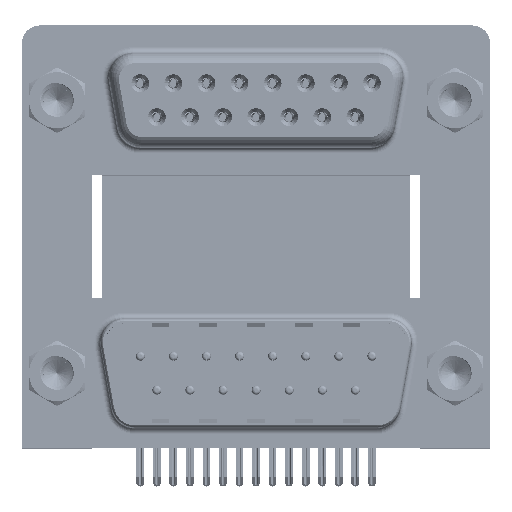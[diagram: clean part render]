
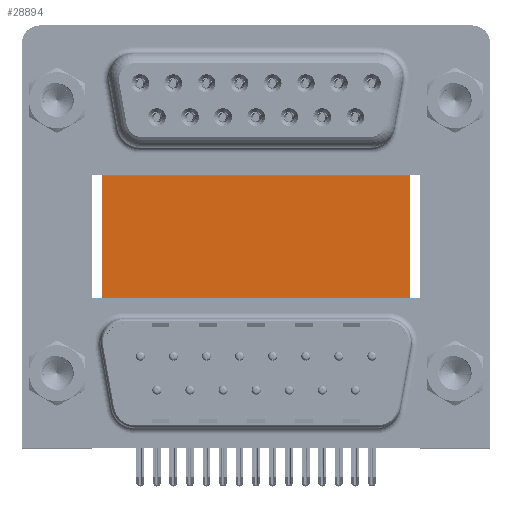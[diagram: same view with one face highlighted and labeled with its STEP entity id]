
A CAD part, top view. The second image highlights one B-rep face of the part: STEP entity #28894.
In plain terms, the highlighted planar face has unit normal (0, 0, 1).
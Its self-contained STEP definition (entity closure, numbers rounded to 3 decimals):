
#5209 = ORIENTED_EDGE ( 'NONE', *, *, #30628, .T. ) ;
#8389 = DIRECTION ( 'NONE',  ( 1., 0., 0. ) ) ;
#11721 = DIRECTION ( 'NONE',  ( 0., 0., -1. ) ) ;
#14759 = VECTOR ( 'NONE', #8389, 1000. ) ;
#15286 = EDGE_CURVE ( 'NONE', #41101, #31572, #44285, .T. ) ;
#15950 = VECTOR ( 'NONE', #24155, 1000. ) ;
#16195 = CARTESIAN_POINT ( 'NONE',  ( 29.58, -3.735, -12. ) ) ;
#16615 = LINE ( 'NONE', #28815, #15950 ) ;
#19431 = VERTEX_POINT ( 'NONE', #50490 ) ;
#20967 = CARTESIAN_POINT ( 'NONE',  ( 3.79, 16.585, -12. ) ) ;
#23330 = LINE ( 'NONE', #51083, #27677 ) ;
#23387 = DIRECTION ( 'NONE',  ( -1., 0., 0. ) ) ;
#23452 = CARTESIAN_POINT ( 'NONE',  ( 3.79, 16.585, -12. ) ) ;
#24155 = DIRECTION ( 'NONE',  ( 0., -1., 0. ) ) ;
#27655 = VERTEX_POINT ( 'NONE', #37978 ) ;
#27677 = VECTOR ( 'NONE', #43553, 1000. ) ;
#28505 = FACE_OUTER_BOUND ( 'NONE', #46814, .T. ) ;
#28815 = CARTESIAN_POINT ( 'NONE',  ( 3.79, 16.585, -12. ) ) ;
#28894 = ADVANCED_FACE ( 'NONE', ( #28505 ), #40937, .F. ) ;
#29231 = DIRECTION ( 'NONE',  ( 1., 0., 0. ) ) ;
#30628 = EDGE_CURVE ( 'NONE', #19431, #41101, #16615, .T. ) ;
#31572 = VERTEX_POINT ( 'NONE', #16195 ) ;
#32853 = CARTESIAN_POINT ( 'NONE',  ( 3.79, -3.735, -12. ) ) ;
#35945 = ORIENTED_EDGE ( 'NONE', *, *, #42750, .F. ) ;
#37017 = AXIS2_PLACEMENT_3D ( 'NONE', #20967, #11721, #23387 ) ;
#37978 = CARTESIAN_POINT ( 'NONE',  ( 29.58, 16.585, -12. ) ) ;
#38406 = CARTESIAN_POINT ( 'NONE',  ( 3.79, -3.735, -12. ) ) ;
#40937 = PLANE ( 'NONE',  #37017 ) ;
#41101 = VERTEX_POINT ( 'NONE', #38406 ) ;
#42750 = EDGE_CURVE ( 'NONE', #27655, #31572, #23330, .T. ) ;
#43156 = LINE ( 'NONE', #23452, #14759 ) ;
#43553 = DIRECTION ( 'NONE',  ( 0., -1., 0. ) ) ;
#44285 = LINE ( 'NONE', #32853, #48628 ) ;
#45251 = ORIENTED_EDGE ( 'NONE', *, *, #50366, .F. ) ;
#46814 = EDGE_LOOP ( 'NONE', ( #49909, #35945, #45251, #5209 ) ) ;
#48628 = VECTOR ( 'NONE', #29231, 1000. ) ;
#49909 = ORIENTED_EDGE ( 'NONE', *, *, #15286, .T. ) ;
#50366 = EDGE_CURVE ( 'NONE', #19431, #27655, #43156, .T. ) ;
#50490 = CARTESIAN_POINT ( 'NONE',  ( 3.79, 16.585, -12. ) ) ;
#51083 = CARTESIAN_POINT ( 'NONE',  ( 29.58, 16.585, -12. ) ) ;
